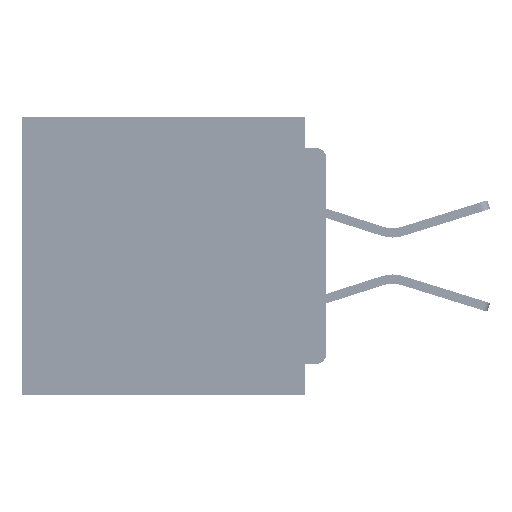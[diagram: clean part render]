
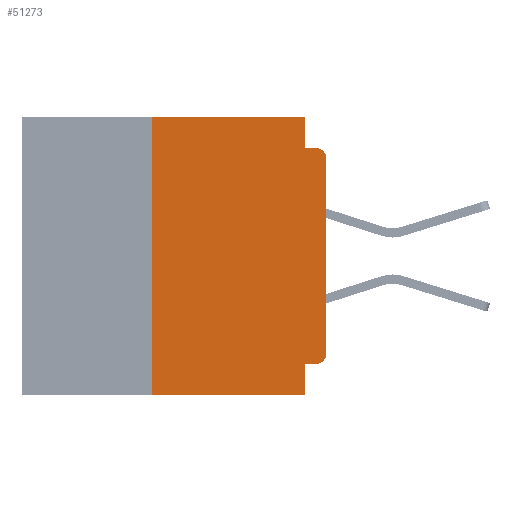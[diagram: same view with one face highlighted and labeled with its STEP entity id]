
A CAD part, left-side view. The second image highlights one B-rep face of the part: STEP entity #51273.
In plain terms, the highlighted planar face has unit normal (-1, 0, 0).
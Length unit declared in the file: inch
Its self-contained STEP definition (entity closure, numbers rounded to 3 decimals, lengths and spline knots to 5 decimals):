
#789 = VECTOR ( 'NONE', #31859, 39.37008 ) ;
#1428 = DIRECTION ( 'NONE',  ( 0., -1., 0. ) ) ;
#1541 = EDGE_CURVE ( 'NONE', #58890, #54786, #16284, .T. ) ;
#1721 = VERTEX_POINT ( 'NONE', #4229 ) ;
#3132 = LINE ( 'NONE', #48705, #28375 ) ;
#3280 = ORIENTED_EDGE ( 'NONE', *, *, #43174, .F. ) ;
#4229 = CARTESIAN_POINT ( 'NONE',  ( 0., 0., -0.06 ) ) ;
#5735 = DIRECTION ( 'NONE',  ( 0., -1., 0. ) ) ;
#6150 = VERTEX_POINT ( 'NONE', #25474 ) ;
#8551 = EDGE_CURVE ( 'NONE', #60331, #64340, #42552, .T. ) ;
#8718 = CARTESIAN_POINT ( 'NONE',  ( 0., 0., -0.355 ) ) ;
#9499 = ORIENTED_EDGE ( 'NONE', *, *, #30075, .F. ) ;
#9690 = VECTOR ( 'NONE', #55591, 39.37008 ) ;
#10003 = EDGE_CURVE ( 'NONE', #60331, #41826, #48227, .T. ) ;
#10037 = CARTESIAN_POINT ( 'NONE',  ( 0., 0.031, 0. ) ) ;
#10595 = LINE ( 'NONE', #10037, #24907 ) ;
#11392 = LINE ( 'NONE', #50223, #9690 ) ;
#11549 = VECTOR ( 'NONE', #62088, 39.37008 ) ;
#12782 = VECTOR ( 'NONE', #1428, 39.37008 ) ;
#13682 = CARTESIAN_POINT ( 'NONE',  ( 0., 0.031, 0. ) ) ;
#15124 = LINE ( 'NONE', #15644, #789 ) ;
#15531 = CARTESIAN_POINT ( 'NONE',  ( 0., 0.015, -0.045 ) ) ;
#15644 = CARTESIAN_POINT ( 'NONE',  ( 0., 0., -0.045 ) ) ;
#15921 = ORIENTED_EDGE ( 'NONE', *, *, #55752, .T. ) ;
#16284 = LINE ( 'NONE', #66724, #28912 ) ;
#17294 = ORIENTED_EDGE ( 'NONE', *, *, #22850, .F. ) ;
#20081 = VERTEX_POINT ( 'NONE', #35815 ) ;
#20748 = DIRECTION ( 'NONE',  ( -1., 0., 0. ) ) ;
#22850 = EDGE_CURVE ( 'NONE', #26337, #6150, #10595, .T. ) ;
#24907 = VECTOR ( 'NONE', #68725, 39.37008 ) ;
#25474 = CARTESIAN_POINT ( 'NONE',  ( 0., 0.031, -0.045 ) ) ;
#26337 = VERTEX_POINT ( 'NONE', #13682 ) ;
#27661 = CARTESIAN_POINT ( 'NONE',  ( 0., 0.031, -0.355 ) ) ;
#28375 = VECTOR ( 'NONE', #5735, 39.37008 ) ;
#28501 = CARTESIAN_POINT ( 'NONE',  ( 0., 0.437, 0. ) ) ;
#28912 = VECTOR ( 'NONE', #66968, 39.37008 ) ;
#28970 = CARTESIAN_POINT ( 'NONE',  ( 0., 0.25, -0.4 ) ) ;
#29304 = CARTESIAN_POINT ( 'NONE',  ( 0., 0., -0.34 ) ) ;
#29378 = CARTESIAN_POINT ( 'NONE',  ( 0., 0.015, -0.06 ) ) ;
#30013 = VECTOR ( 'NONE', #51659, 39.37008 ) ;
#30075 = EDGE_CURVE ( 'NONE', #54786, #26337, #3132, .T. ) ;
#31622 = EDGE_CURVE ( 'NONE', #1721, #63623, #43243, .T. ) ;
#31859 = DIRECTION ( 'NONE',  ( 0., -1., 0. ) ) ;
#33487 = AXIS2_PLACEMENT_3D ( 'NONE', #29378, #66659, #34780 ) ;
#33924 = DIRECTION ( 'NONE',  ( 0., 0., -1. ) ) ;
#34780 = DIRECTION ( 'NONE',  ( 0., 0., -1. ) ) ;
#35815 = CARTESIAN_POINT ( 'NONE',  ( 0., 0.031, -0.4 ) ) ;
#38217 = AXIS2_PLACEMENT_3D ( 'NONE', #28501, #65807, #33924 ) ;
#38451 = EDGE_CURVE ( 'NONE', #64340, #20081, #56015, .T. ) ;
#39345 = AXIS2_PLACEMENT_3D ( 'NONE', #52880, #20748, #58211 ) ;
#40844 = ORIENTED_EDGE ( 'NONE', *, *, #8551, .F. ) ;
#41826 = VERTEX_POINT ( 'NONE', #29304 ) ;
#42552 = LINE ( 'NONE', #8718, #30013 ) ;
#43174 = EDGE_CURVE ( 'NONE', #6150, #63623, #15124, .T. ) ;
#43243 = CIRCLE ( 'NONE', #33487, 0.015 ) ;
#46794 = ORIENTED_EDGE ( 'NONE', *, *, #1541, .F. ) ;
#48227 = CIRCLE ( 'NONE', #39345, 0.015 ) ;
#48705 = CARTESIAN_POINT ( 'NONE',  ( 0., 0.437, 0. ) ) ;
#48842 = ORIENTED_EDGE ( 'NONE', *, *, #10003, .T. ) ;
#49176 = EDGE_LOOP ( 'NONE', ( #15921, #59210, #3280, #17294, #9499, #46794, #63421, #49639, #40844, #48842 ) ) ;
#49639 = ORIENTED_EDGE ( 'NONE', *, *, #38451, .F. ) ;
#50223 = CARTESIAN_POINT ( 'NONE',  ( 0., 0., 0. ) ) ;
#51250 = EDGE_CURVE ( 'NONE', #58890, #20081, #55573, .T. ) ;
#51273 = ADVANCED_FACE ( 'NONE', ( #53923 ), #60492, .F. ) ;
#51659 = DIRECTION ( 'NONE',  ( 0., 1., 0. ) ) ;
#52473 = CARTESIAN_POINT ( 'NONE',  ( 0., 0.25, 0. ) ) ;
#52880 = CARTESIAN_POINT ( 'NONE',  ( 0., 0.015, -0.34 ) ) ;
#53923 = FACE_OUTER_BOUND ( 'NONE', #49176, .T. ) ;
#54786 = VERTEX_POINT ( 'NONE', #52473 ) ;
#54948 = CARTESIAN_POINT ( 'NONE',  ( 0., 0.437, -0.4 ) ) ;
#55573 = LINE ( 'NONE', #54948, #12782 ) ;
#55591 = DIRECTION ( 'NONE',  ( 0., 0., 1. ) ) ;
#55752 = EDGE_CURVE ( 'NONE', #41826, #1721, #11392, .T. ) ;
#56015 = LINE ( 'NONE', #67384, #11549 ) ;
#58211 = DIRECTION ( 'NONE',  ( 0., 0., -1. ) ) ;
#58890 = VERTEX_POINT ( 'NONE', #28970 ) ;
#59210 = ORIENTED_EDGE ( 'NONE', *, *, #31622, .T. ) ;
#60331 = VERTEX_POINT ( 'NONE', #63546 ) ;
#60492 = PLANE ( 'NONE',  #38217 ) ;
#62088 = DIRECTION ( 'NONE',  ( 0., 0., -1. ) ) ;
#63421 = ORIENTED_EDGE ( 'NONE', *, *, #51250, .T. ) ;
#63546 = CARTESIAN_POINT ( 'NONE',  ( 0., 0.015, -0.355 ) ) ;
#63623 = VERTEX_POINT ( 'NONE', #15531 ) ;
#64340 = VERTEX_POINT ( 'NONE', #27661 ) ;
#65807 = DIRECTION ( 'NONE',  ( 1., 0., 0. ) ) ;
#66659 = DIRECTION ( 'NONE',  ( -1., 0., 0. ) ) ;
#66724 = CARTESIAN_POINT ( 'NONE',  ( 0., 0.25, -0.4 ) ) ;
#66968 = DIRECTION ( 'NONE',  ( 0., 0., 1. ) ) ;
#67384 = CARTESIAN_POINT ( 'NONE',  ( 0., 0.031, -0.4 ) ) ;
#68725 = DIRECTION ( 'NONE',  ( 0., 0., -1. ) ) ;
